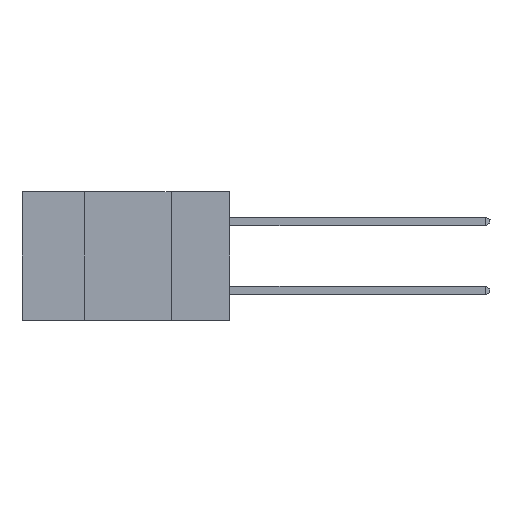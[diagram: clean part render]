
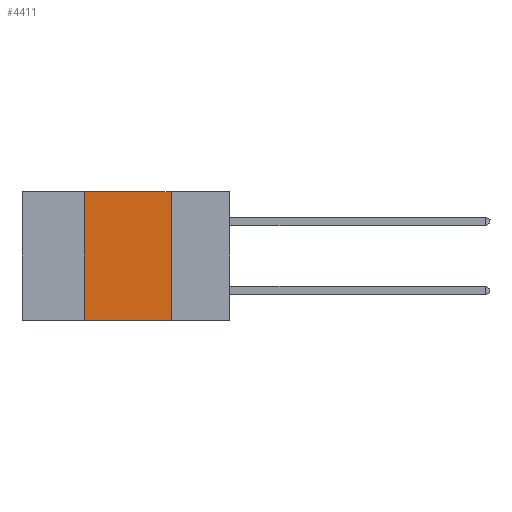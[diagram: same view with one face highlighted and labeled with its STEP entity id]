
A CAD part, left-side view. The second image highlights one B-rep face of the part: STEP entity #4411.
In plain terms, the highlighted planar face has unit normal (-1, 0, 0).
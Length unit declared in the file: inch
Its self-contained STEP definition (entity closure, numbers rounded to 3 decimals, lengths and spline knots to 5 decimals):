
#242 = CARTESIAN_POINT ( 'NONE',  ( 0., 0.42, -0.37 ) ) ;
#371 = LINE ( 'NONE', #7769, #8292 ) ;
#530 = EDGE_CURVE ( 'NONE', #4880, #5622, #371, .T. ) ;
#1099 = VECTOR ( 'NONE', #5170, 39.37008 ) ;
#1221 = VECTOR ( 'NONE', #7632, 39.37008 ) ;
#1447 = CARTESIAN_POINT ( 'NONE',  ( 0., 0.17, 0. ) ) ;
#1646 = VERTEX_POINT ( 'NONE', #4388 ) ;
#1913 = ORIENTED_EDGE ( 'NONE', *, *, #7674, .F. ) ;
#1964 = EDGE_CURVE ( 'NONE', #6920, #5622, #7325, .T. ) ;
#3231 = CARTESIAN_POINT ( 'NONE',  ( 0., 0.42, 0. ) ) ;
#3320 = CARTESIAN_POINT ( 'NONE',  ( 0., 0.17, 0. ) ) ;
#3492 = EDGE_CURVE ( 'NONE', #4880, #1646, #7675, .T. ) ;
#3573 = PLANE ( 'NONE',  #7412 ) ;
#4388 = CARTESIAN_POINT ( 'NONE',  ( 0., 0.42, 0. ) ) ;
#4411 = ADVANCED_FACE ( 'NONE', ( #9573 ), #3573, .F. ) ;
#4880 = VERTEX_POINT ( 'NONE', #242 ) ;
#4926 = LINE ( 'NONE', #9104, #1099 ) ;
#5005 = VECTOR ( 'NONE', #5856, 39.37008 ) ;
#5060 = ORIENTED_EDGE ( 'NONE', *, *, #1964, .F. ) ;
#5170 = DIRECTION ( 'NONE',  ( 0., -1., 0. ) ) ;
#5286 = DIRECTION ( 'NONE',  ( 0., -1., 0. ) ) ;
#5489 = ORIENTED_EDGE ( 'NONE', *, *, #530, .T. ) ;
#5622 = VERTEX_POINT ( 'NONE', #7020 ) ;
#5856 = DIRECTION ( 'NONE',  ( 0., 0., 1. ) ) ;
#6920 = VERTEX_POINT ( 'NONE', #1447 ) ;
#6933 = DIRECTION ( 'NONE',  ( 1., 0., 0. ) ) ;
#7020 = CARTESIAN_POINT ( 'NONE',  ( 0., 0.17, -0.37 ) ) ;
#7261 = EDGE_LOOP ( 'NONE', ( #5060, #1913, #7618, #5489 ) ) ;
#7325 = LINE ( 'NONE', #3320, #1221 ) ;
#7412 = AXIS2_PLACEMENT_3D ( 'NONE', #9371, #6933, #7755 ) ;
#7618 = ORIENTED_EDGE ( 'NONE', *, *, #3492, .F. ) ;
#7632 = DIRECTION ( 'NONE',  ( 0., 0., -1. ) ) ;
#7674 = EDGE_CURVE ( 'NONE', #1646, #6920, #4926, .T. ) ;
#7675 = LINE ( 'NONE', #3231, #5005 ) ;
#7755 = DIRECTION ( 'NONE',  ( 0., 0., -1. ) ) ;
#7769 = CARTESIAN_POINT ( 'NONE',  ( 0., 0.6, -0.37 ) ) ;
#8292 = VECTOR ( 'NONE', #5286, 39.37008 ) ;
#9104 = CARTESIAN_POINT ( 'NONE',  ( 0., 0.6, 0. ) ) ;
#9371 = CARTESIAN_POINT ( 'NONE',  ( 0., 0.6, 0. ) ) ;
#9573 = FACE_OUTER_BOUND ( 'NONE', #7261, .T. ) ;
